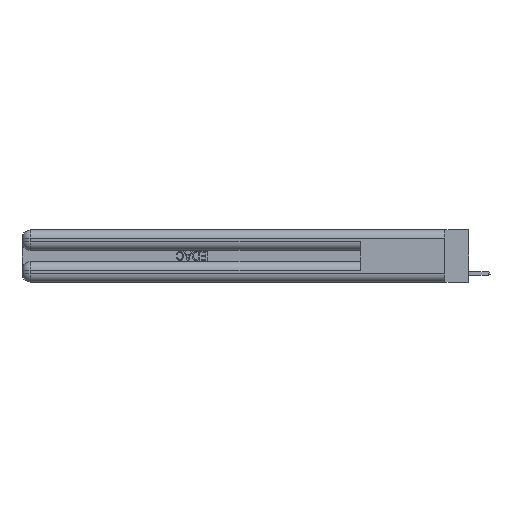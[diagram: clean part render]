
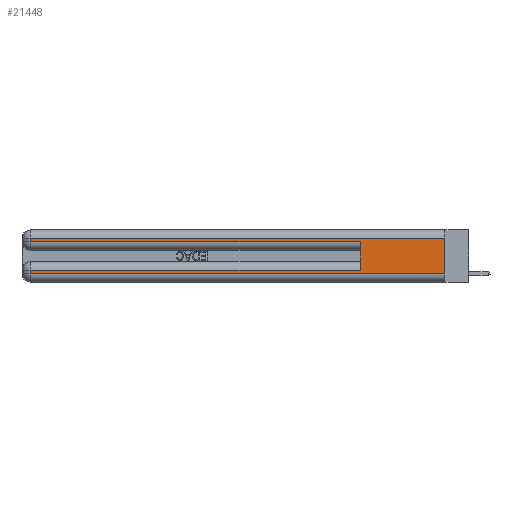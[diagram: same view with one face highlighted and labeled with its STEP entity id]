
A CAD part, left-side view. The second image highlights one B-rep face of the part: STEP entity #21448.
In plain terms, the highlighted planar face has unit normal (-1, 0, 0).
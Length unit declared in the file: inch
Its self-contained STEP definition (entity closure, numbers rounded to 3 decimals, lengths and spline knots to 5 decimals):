
#54 = ORIENTED_EDGE ( 'NONE', *, *, #3031, .F. ) ;
#602 = DIRECTION ( 'NONE',  ( 0., 0., -1. ) ) ;
#915 = VERTEX_POINT ( 'NONE', #5680 ) ;
#1109 = LINE ( 'NONE', #9488, #1558 ) ;
#1152 = VERTEX_POINT ( 'NONE', #9918 ) ;
#1558 = VECTOR ( 'NONE', #18229, 39.37008 ) ;
#2337 = CARTESIAN_POINT ( 'NONE',  ( 0., 0., 0.37 ) ) ;
#2457 = LINE ( 'NONE', #19710, #15726 ) ;
#2554 = VECTOR ( 'NONE', #14896, 39.37008 ) ;
#2590 = EDGE_CURVE ( 'NONE', #915, #2759, #2821, .T. ) ;
#2759 = VERTEX_POINT ( 'NONE', #24383 ) ;
#2821 = LINE ( 'NONE', #18918, #2554 ) ;
#2857 = ORIENTED_EDGE ( 'NONE', *, *, #2590, .T. ) ;
#3031 = EDGE_CURVE ( 'NONE', #3248, #27980, #19428, .T. ) ;
#3248 = VERTEX_POINT ( 'NONE', #24724 ) ;
#3280 = ORIENTED_EDGE ( 'NONE', *, *, #6742, .T. ) ;
#3504 = DIRECTION ( 'NONE',  ( 0., 0., 1. ) ) ;
#3763 = DIRECTION ( 'NONE',  ( 0., -1., 0. ) ) ;
#4326 = ORIENTED_EDGE ( 'NONE', *, *, #9381, .T. ) ;
#4357 = DIRECTION ( 'NONE',  ( 0., 1., 0. ) ) ;
#5680 = CARTESIAN_POINT ( 'NONE',  ( 0., 2.94, 0.06 ) ) ;
#6114 = CARTESIAN_POINT ( 'NONE',  ( 0., 0.6, 0.285 ) ) ;
#6142 = EDGE_LOOP ( 'NONE', ( #22881, #3280, #12395, #28327, #54, #4326, #6758, #2857 ) ) ;
#6210 = CARTESIAN_POINT ( 'NONE',  ( 0., 0.6, 0.145 ) ) ;
#6742 = EDGE_CURVE ( 'NONE', #20999, #1152, #17508, .T. ) ;
#6746 = DIRECTION ( 'NONE',  ( 0., 1., 0. ) ) ;
#6758 = ORIENTED_EDGE ( 'NONE', *, *, #24422, .T. ) ;
#8017 = VECTOR ( 'NONE', #3763, 39.37008 ) ;
#8216 = CARTESIAN_POINT ( 'NONE',  ( 0., 0., 0.285 ) ) ;
#8775 = CARTESIAN_POINT ( 'NONE',  ( 0., 2.94, 0.085 ) ) ;
#9381 = EDGE_CURVE ( 'NONE', #3248, #10908, #2457, .T. ) ;
#9488 = CARTESIAN_POINT ( 'NONE',  ( 0., 2.94, 0.37 ) ) ;
#9918 = CARTESIAN_POINT ( 'NONE',  ( 0., 2.94, 0.31 ) ) ;
#10908 = VERTEX_POINT ( 'NONE', #8775 ) ;
#11141 = DIRECTION ( 'NONE',  ( 1., 0., 0. ) ) ;
#12027 = VECTOR ( 'NONE', #6746, 39.37008 ) ;
#12395 = ORIENTED_EDGE ( 'NONE', *, *, #16079, .T. ) ;
#13230 = VECTOR ( 'NONE', #24022, 39.37008 ) ;
#14165 = CARTESIAN_POINT ( 'NONE',  ( 0., 0., 0.31 ) ) ;
#14604 = EDGE_CURVE ( 'NONE', #20725, #27980, #16957, .T. ) ;
#14896 = DIRECTION ( 'NONE',  ( 0., -1., 0. ) ) ;
#14950 = LINE ( 'NONE', #17509, #13230 ) ;
#15043 = CARTESIAN_POINT ( 'NONE',  ( 0., 2.94, 0.285 ) ) ;
#15577 = LINE ( 'NONE', #24911, #18457 ) ;
#15726 = VECTOR ( 'NONE', #4357, 39.37008 ) ;
#16079 = EDGE_CURVE ( 'NONE', #1152, #20725, #1109, .T. ) ;
#16957 = LINE ( 'NONE', #8216, #8017 ) ;
#17508 = LINE ( 'NONE', #14165, #12027 ) ;
#17509 = CARTESIAN_POINT ( 'NONE',  ( 0., 2.94, 0.37 ) ) ;
#17718 = DIRECTION ( 'NONE',  ( 0., 0., -1. ) ) ;
#18229 = DIRECTION ( 'NONE',  ( 0., 0., -1. ) ) ;
#18457 = VECTOR ( 'NONE', #602, 39.37008 ) ;
#18918 = CARTESIAN_POINT ( 'NONE',  ( 0., 0., 0.06 ) ) ;
#19428 = LINE ( 'NONE', #6210, #19578 ) ;
#19578 = VECTOR ( 'NONE', #3504, 39.37008 ) ;
#19710 = CARTESIAN_POINT ( 'NONE',  ( 0., 0., 0.085 ) ) ;
#20468 = CARTESIAN_POINT ( 'NONE',  ( 0., 0., 0.31 ) ) ;
#20725 = VERTEX_POINT ( 'NONE', #15043 ) ;
#20999 = VERTEX_POINT ( 'NONE', #20468 ) ;
#21448 = ADVANCED_FACE ( 'NONE', ( #22047 ), #24354, .F. ) ;
#22047 = FACE_OUTER_BOUND ( 'NONE', #6142, .T. ) ;
#22523 = EDGE_CURVE ( 'NONE', #20999, #2759, #15577, .T. ) ;
#22881 = ORIENTED_EDGE ( 'NONE', *, *, #22523, .F. ) ;
#24022 = DIRECTION ( 'NONE',  ( 0., 0., -1. ) ) ;
#24354 = PLANE ( 'NONE',  #26293 ) ;
#24383 = CARTESIAN_POINT ( 'NONE',  ( 0., 0., 0.06 ) ) ;
#24422 = EDGE_CURVE ( 'NONE', #10908, #915, #14950, .T. ) ;
#24724 = CARTESIAN_POINT ( 'NONE',  ( 0., 0.6, 0.085 ) ) ;
#24911 = CARTESIAN_POINT ( 'NONE',  ( 0., 0., 0.37 ) ) ;
#26293 = AXIS2_PLACEMENT_3D ( 'NONE', #2337, #11141, #17718 ) ;
#27980 = VERTEX_POINT ( 'NONE', #6114 ) ;
#28327 = ORIENTED_EDGE ( 'NONE', *, *, #14604, .T. ) ;
